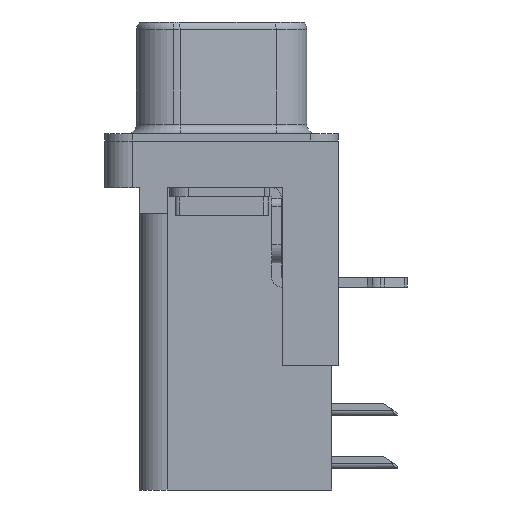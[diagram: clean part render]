
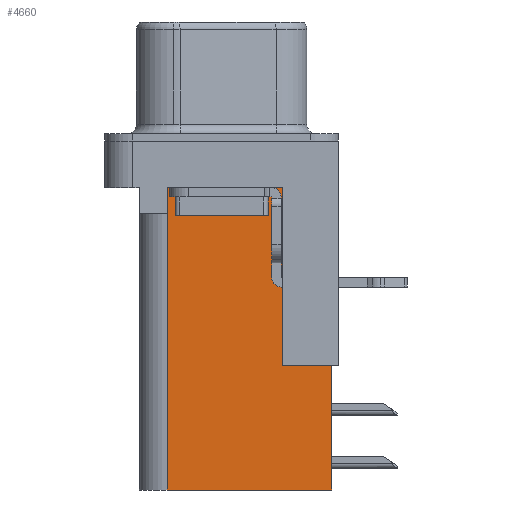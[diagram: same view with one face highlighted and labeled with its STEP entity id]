
A CAD part, left-side view. The second image highlights one B-rep face of the part: STEP entity #4660.
In plain terms, the highlighted planar face has unit normal (-1, 0, 0).
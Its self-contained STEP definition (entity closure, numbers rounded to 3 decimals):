
#68 = DIRECTION ( 'NONE',  ( 0., 0., 1. ) ) ;
#124 = VERTEX_POINT ( 'NONE', #16890 ) ;
#488 = DIRECTION ( 'NONE',  ( 0., 1., 0. ) ) ;
#615 = ORIENTED_EDGE ( 'NONE', *, *, #12769, .T. ) ;
#1265 = VECTOR ( 'NONE', #8610, 1000. ) ;
#1945 = LINE ( 'NONE', #9062, #18189 ) ;
#2273 = LINE ( 'NONE', #9183, #18991 ) ;
#2419 = VECTOR ( 'NONE', #19751, 1000. ) ;
#2612 = CARTESIAN_POINT ( 'NONE',  ( 3.765, 2.895, -2.5 ) ) ;
#2987 = ORIENTED_EDGE ( 'NONE', *, *, #12740, .F. ) ;
#3225 = ORIENTED_EDGE ( 'NONE', *, *, #17653, .T. ) ;
#3684 = LINE ( 'NONE', #11004, #7183 ) ;
#4372 = DIRECTION ( 'NONE',  ( 0., 0., -1. ) ) ;
#4408 = CARTESIAN_POINT ( 'NONE',  ( 3.765, -5.925, -18.76 ) ) ;
#4430 = CARTESIAN_POINT ( 'NONE',  ( 3.765, -5.925, -2. ) ) ;
#4660 = ADVANCED_FACE ( 'NONE', ( #12444 ), #16679, .F. ) ;
#5297 = VERTEX_POINT ( 'NONE', #14180 ) ;
#5973 = VECTOR ( 'NONE', #17862, 1000. ) ;
#6164 = CARTESIAN_POINT ( 'NONE',  ( 3.765, -3.295, -18.76 ) ) ;
#6234 = DIRECTION ( 'NONE',  ( 1., 0., 0. ) ) ;
#6848 = LINE ( 'NONE', #16642, #7307 ) ;
#7183 = VECTOR ( 'NONE', #488, 1000. ) ;
#7307 = VECTOR ( 'NONE', #7377, 1000. ) ;
#7377 = DIRECTION ( 'NONE',  ( 0., 1., 0. ) ) ;
#7466 = CARTESIAN_POINT ( 'NONE',  ( 3.765, -3.295, -2.5 ) ) ;
#8571 = DIRECTION ( 'NONE',  ( 0., 1., 0. ) ) ;
#8610 = DIRECTION ( 'NONE',  ( 0., 0., 1. ) ) ;
#9062 = CARTESIAN_POINT ( 'NONE',  ( 3.765, -3.295, -18.76 ) ) ;
#9183 = CARTESIAN_POINT ( 'NONE',  ( 3.765, 0., -3.9 ) ) ;
#10170 = VERTEX_POINT ( 'NONE', #13206 ) ;
#10435 = VECTOR ( 'NONE', #4372, 1000. ) ;
#10751 = VERTEX_POINT ( 'NONE', #12988 ) ;
#10849 = VERTEX_POINT ( 'NONE', #2612 ) ;
#11004 = CARTESIAN_POINT ( 'NONE',  ( 3.765, -3.295, -2.5 ) ) ;
#11530 = AXIS2_PLACEMENT_3D ( 'NONE', #6164, #6234, #8571 ) ;
#12444 = FACE_OUTER_BOUND ( 'NONE', #15693, .T. ) ;
#12623 = EDGE_CURVE ( 'NONE', #10751, #17141, #13356, .T. ) ;
#12691 = ORIENTED_EDGE ( 'NONE', *, *, #18219, .T. ) ;
#12719 = EDGE_CURVE ( 'NONE', #13183, #10751, #6848, .T. ) ;
#12740 = EDGE_CURVE ( 'NONE', #10170, #13183, #15544, .T. ) ;
#12743 = EDGE_CURVE ( 'NONE', #10170, #124, #14572, .T. ) ;
#12769 = EDGE_CURVE ( 'NONE', #124, #19192, #1945, .T. ) ;
#12774 = ORIENTED_EDGE ( 'NONE', *, *, #12623, .F. ) ;
#12988 = CARTESIAN_POINT ( 'NONE',  ( 3.765, 2.925, -18.76 ) ) ;
#13183 = VERTEX_POINT ( 'NONE', #4408 ) ;
#13206 = CARTESIAN_POINT ( 'NONE',  ( 3.765, -5.925, -12.05 ) ) ;
#13356 = LINE ( 'NONE', #16314, #1265 ) ;
#13835 = DIRECTION ( 'NONE',  ( 0., 1., 0. ) ) ;
#14180 = CARTESIAN_POINT ( 'NONE',  ( 3.765, 2.895, -3.9 ) ) ;
#14572 = LINE ( 'NONE', #18260, #2419 ) ;
#14591 = ORIENTED_EDGE ( 'NONE', *, *, #17923, .T. ) ;
#15544 = LINE ( 'NONE', #4430, #10435 ) ;
#15693 = EDGE_LOOP ( 'NONE', ( #3225, #14591, #12691, #12774, #16523, #2987, #17793, #615 ) ) ;
#16301 = CARTESIAN_POINT ( 'NONE',  ( 3.765, 2.895, -3.9 ) ) ;
#16314 = CARTESIAN_POINT ( 'NONE',  ( 3.765, 2.925, -18.76 ) ) ;
#16523 = ORIENTED_EDGE ( 'NONE', *, *, #12719, .F. ) ;
#16642 = CARTESIAN_POINT ( 'NONE',  ( 3.765, -3.295, -18.76 ) ) ;
#16679 = PLANE ( 'NONE',  #11530 ) ;
#16890 = CARTESIAN_POINT ( 'NONE',  ( 3.765, -3.295, -12.05 ) ) ;
#17141 = VERTEX_POINT ( 'NONE', #17543 ) ;
#17543 = CARTESIAN_POINT ( 'NONE',  ( 3.765, 2.925, -3.9 ) ) ;
#17653 = EDGE_CURVE ( 'NONE', #19192, #10849, #3684, .T. ) ;
#17793 = ORIENTED_EDGE ( 'NONE', *, *, #12743, .T. ) ;
#17862 = DIRECTION ( 'NONE',  ( 0., 0., -1. ) ) ;
#17923 = EDGE_CURVE ( 'NONE', #10849, #5297, #18290, .T. ) ;
#18189 = VECTOR ( 'NONE', #68, 1000. ) ;
#18219 = EDGE_CURVE ( 'NONE', #5297, #17141, #2273, .T. ) ;
#18260 = CARTESIAN_POINT ( 'NONE',  ( 3.765, -6.295, -12.05 ) ) ;
#18290 = LINE ( 'NONE', #16301, #5973 ) ;
#18991 = VECTOR ( 'NONE', #13835, 1000. ) ;
#19192 = VERTEX_POINT ( 'NONE', #7466 ) ;
#19751 = DIRECTION ( 'NONE',  ( 0., 1., 0. ) ) ;
